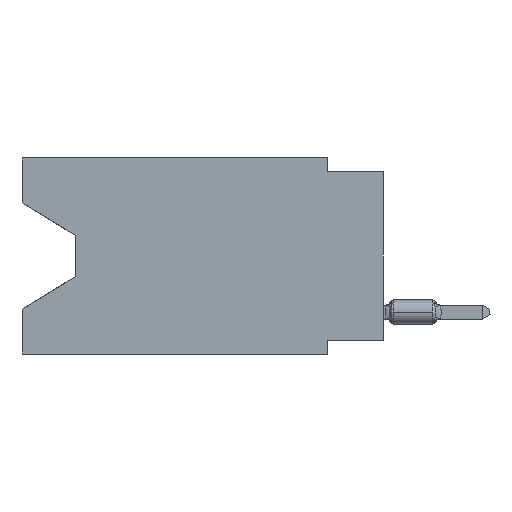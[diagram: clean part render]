
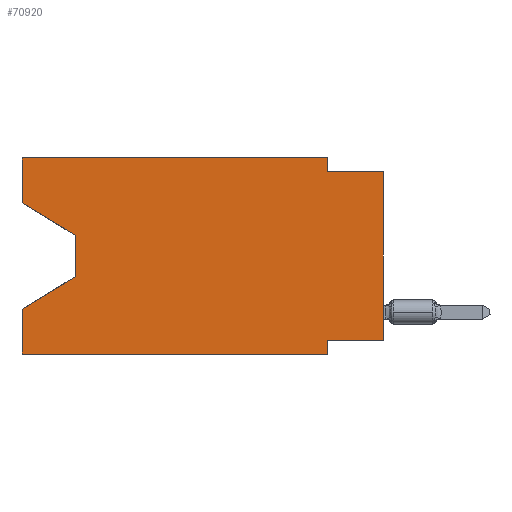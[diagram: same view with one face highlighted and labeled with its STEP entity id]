
A CAD part, left-side view. The second image highlights one B-rep face of the part: STEP entity #70920.
In plain terms, the highlighted planar face has unit normal (-1, 0, 0).
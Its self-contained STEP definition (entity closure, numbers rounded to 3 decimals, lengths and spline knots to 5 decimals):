
#303 = DIRECTION ( 'NONE',  ( 0., 0., -1. ) ) ;
#1064 = ORIENTED_EDGE ( 'NONE', *, *, #35114, .F. ) ;
#1827 = DIRECTION ( 'NONE',  ( 0., -1., 0. ) ) ;
#2335 = VERTEX_POINT ( 'NONE', #81327 ) ;
#5913 = LINE ( 'NONE', #32441, #8033 ) ;
#6395 = FACE_OUTER_BOUND ( 'NONE', #60324, .T. ) ;
#6553 = LINE ( 'NONE', #73124, #24607 ) ;
#7330 = CARTESIAN_POINT ( 'NONE',  ( 0., 0.645, 0. ) ) ;
#7757 = VECTOR ( 'NONE', #13437, 39.37008 ) ;
#8033 = VECTOR ( 'NONE', #58997, 39.37008 ) ;
#8582 = CARTESIAN_POINT ( 'NONE',  ( 0., 0., 0. ) ) ;
#8603 = CARTESIAN_POINT ( 'NONE',  ( 0., 0., -0.025 ) ) ;
#10686 = ORIENTED_EDGE ( 'NONE', *, *, #65434, .T. ) ;
#11781 = DIRECTION ( 'NONE',  ( 0., 0., 1. ) ) ;
#12854 = ORIENTED_EDGE ( 'NONE', *, *, #21877, .F. ) ;
#13042 = ORIENTED_EDGE ( 'NONE', *, *, #28997, .T. ) ;
#13437 = DIRECTION ( 'NONE',  ( 0., -1., 0. ) ) ;
#15532 = DIRECTION ( 'NONE',  ( 0., 0., 1. ) ) ;
#15606 = ORIENTED_EDGE ( 'NONE', *, *, #67352, .F. ) ;
#15863 = DIRECTION ( 'NONE',  ( 0., 0., -1. ) ) ;
#19024 = CARTESIAN_POINT ( 'NONE',  ( 0., 0.645, 0. ) ) ;
#19067 = DIRECTION ( 'NONE',  ( 0., -1., 0. ) ) ;
#20027 = VECTOR ( 'NONE', #30509, 39.37008 ) ;
#21002 = EDGE_CURVE ( 'NONE', #59328, #72239, #6553, .T. ) ;
#21369 = CARTESIAN_POINT ( 'NONE',  ( 0., 0.645, 0. ) ) ;
#21877 = EDGE_CURVE ( 'NONE', #62199, #2335, #5913, .T. ) ;
#22252 = DIRECTION ( 'NONE',  ( 0., 0., -1. ) ) ;
#23074 = VERTEX_POINT ( 'NONE', #51197 ) ;
#23177 = ORIENTED_EDGE ( 'NONE', *, *, #31386, .F. ) ;
#24607 = VECTOR ( 'NONE', #11781, 39.37008 ) ;
#25757 = ORIENTED_EDGE ( 'NONE', *, *, #45930, .F. ) ;
#26406 = DIRECTION ( 'NONE',  ( 1., 0., 0. ) ) ;
#26449 = CARTESIAN_POINT ( 'NONE',  ( 0., 0.645, -0.35 ) ) ;
#26968 = VECTOR ( 'NONE', #19067, 39.37008 ) ;
#27632 = VECTOR ( 'NONE', #15532, 39.37008 ) ;
#28050 = ORIENTED_EDGE ( 'NONE', *, *, #38183, .T. ) ;
#28216 = VECTOR ( 'NONE', #71607, 39.37008 ) ;
#28366 = CARTESIAN_POINT ( 'NONE',  ( 0., 0., -0.325 ) ) ;
#28997 = EDGE_CURVE ( 'NONE', #76944, #72239, #55655, .T. ) ;
#30509 = DIRECTION ( 'NONE',  ( 0., 0., -1. ) ) ;
#30831 = DIRECTION ( 'NONE',  ( 0., 0., 1. ) ) ;
#31386 = EDGE_CURVE ( 'NONE', #65257, #68687, #64750, .T. ) ;
#32441 = CARTESIAN_POINT ( 'NONE',  ( 0., 0., -0.325 ) ) ;
#34181 = CARTESIAN_POINT ( 'NONE',  ( 0., 0.1, 0. ) ) ;
#34455 = CARTESIAN_POINT ( 'NONE',  ( 0., 0., -0.025 ) ) ;
#35114 = EDGE_CURVE ( 'NONE', #45244, #46651, #49201, .T. ) ;
#37076 = EDGE_CURVE ( 'NONE', #62199, #46651, #74296, .T. ) ;
#38183 = EDGE_CURVE ( 'NONE', #59328, #82449, #79973, .T. ) ;
#38326 = LINE ( 'NONE', #57058, #20027 ) ;
#40004 = VECTOR ( 'NONE', #15863, 39.37008 ) ;
#41091 = ORIENTED_EDGE ( 'NONE', *, *, #37076, .T. ) ;
#41735 = EDGE_CURVE ( 'NONE', #65257, #67751, #66265, .T. ) ;
#45069 = CARTESIAN_POINT ( 'NONE',  ( 0., 0.55, -0.212 ) ) ;
#45244 = VERTEX_POINT ( 'NONE', #85777 ) ;
#45930 = EDGE_CURVE ( 'NONE', #23074, #45244, #54204, .T. ) ;
#46390 = CARTESIAN_POINT ( 'NONE',  ( 0., 0.55, -0.138 ) ) ;
#46651 = VERTEX_POINT ( 'NONE', #8603 ) ;
#48416 = CARTESIAN_POINT ( 'NONE',  ( 0., 0.645, -0.08025 ) ) ;
#48486 = VECTOR ( 'NONE', #22252, 39.37008 ) ;
#49201 = LINE ( 'NONE', #34455, #62103 ) ;
#49306 = VECTOR ( 'NONE', #30831, 39.37008 ) ;
#51197 = CARTESIAN_POINT ( 'NONE',  ( 0., 0.1, 0. ) ) ;
#52077 = PLANE ( 'NONE',  #82996 ) ;
#54204 = LINE ( 'NONE', #34181, #40004 ) ;
#55068 = CARTESIAN_POINT ( 'NONE',  ( 0., 0.55, -0.212 ) ) ;
#55655 = LINE ( 'NONE', #45069, #28216 ) ;
#57058 = CARTESIAN_POINT ( 'NONE',  ( 0., 0.55, -0.138 ) ) ;
#58997 = DIRECTION ( 'NONE',  ( 0., 1., 0. ) ) ;
#59328 = VERTEX_POINT ( 'NONE', #76626 ) ;
#60324 = EDGE_LOOP ( 'NONE', ( #72211, #10686, #13042, #71866, #28050, #82327, #12854, #41091, #1064, #25757, #15606, #23177 ) ) ;
#60400 = CARTESIAN_POINT ( 'NONE',  ( 0., 0.645, -0.08025 ) ) ;
#62103 = VECTOR ( 'NONE', #1827, 39.37008 ) ;
#62199 = VERTEX_POINT ( 'NONE', #28366 ) ;
#64022 = LINE ( 'NONE', #7330, #7757 ) ;
#64750 = LINE ( 'NONE', #83928, #49306 ) ;
#65165 = CARTESIAN_POINT ( 'NONE',  ( 0., 0.1, -0.35 ) ) ;
#65257 = VERTEX_POINT ( 'NONE', #60400 ) ;
#65434 = EDGE_CURVE ( 'NONE', #67751, #76944, #38326, .T. ) ;
#66265 = LINE ( 'NONE', #48416, #81393 ) ;
#67352 = EDGE_CURVE ( 'NONE', #68687, #23074, #64022, .T. ) ;
#67751 = VERTEX_POINT ( 'NONE', #46390 ) ;
#67841 = CARTESIAN_POINT ( 'NONE',  ( 0., 0.645, -0.26975 ) ) ;
#68687 = VERTEX_POINT ( 'NONE', #21369 ) ;
#70920 = ADVANCED_FACE ( 'NONE', ( #6395 ), #52077, .F. ) ;
#71607 = DIRECTION ( 'NONE',  ( 0., 0.855, -0.519 ) ) ;
#71866 = ORIENTED_EDGE ( 'NONE', *, *, #21002, .F. ) ;
#72211 = ORIENTED_EDGE ( 'NONE', *, *, #41735, .T. ) ;
#72239 = VERTEX_POINT ( 'NONE', #67841 ) ;
#73124 = CARTESIAN_POINT ( 'NONE',  ( 0., 0.645, 0. ) ) ;
#73128 = EDGE_CURVE ( 'NONE', #2335, #82449, #81858, .T. ) ;
#74296 = LINE ( 'NONE', #8582, #27632 ) ;
#76626 = CARTESIAN_POINT ( 'NONE',  ( 0., 0.645, -0.35 ) ) ;
#76944 = VERTEX_POINT ( 'NONE', #55068 ) ;
#79973 = LINE ( 'NONE', #26449, #26968 ) ;
#80185 = DIRECTION ( 'NONE',  ( 0., -0.855, -0.519 ) ) ;
#80594 = CARTESIAN_POINT ( 'NONE',  ( 0., 0.1, -0.35 ) ) ;
#81327 = CARTESIAN_POINT ( 'NONE',  ( 0., 0.1, -0.325 ) ) ;
#81393 = VECTOR ( 'NONE', #80185, 39.37008 ) ;
#81858 = LINE ( 'NONE', #80594, #48486 ) ;
#82327 = ORIENTED_EDGE ( 'NONE', *, *, #73128, .F. ) ;
#82449 = VERTEX_POINT ( 'NONE', #65165 ) ;
#82996 = AXIS2_PLACEMENT_3D ( 'NONE', #19024, #26406, #303 ) ;
#83928 = CARTESIAN_POINT ( 'NONE',  ( 0., 0.645, 0. ) ) ;
#85777 = CARTESIAN_POINT ( 'NONE',  ( 0., 0.1, -0.025 ) ) ;
